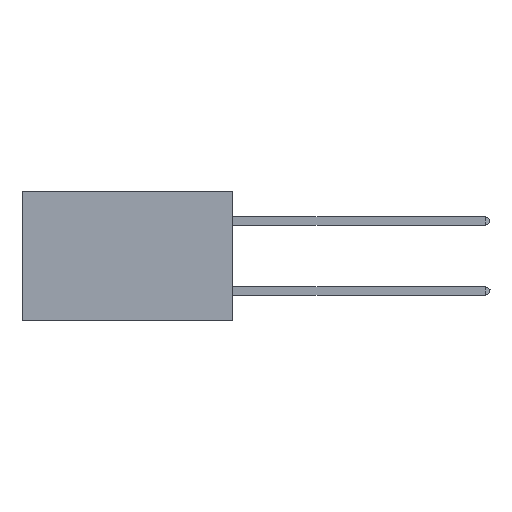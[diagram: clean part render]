
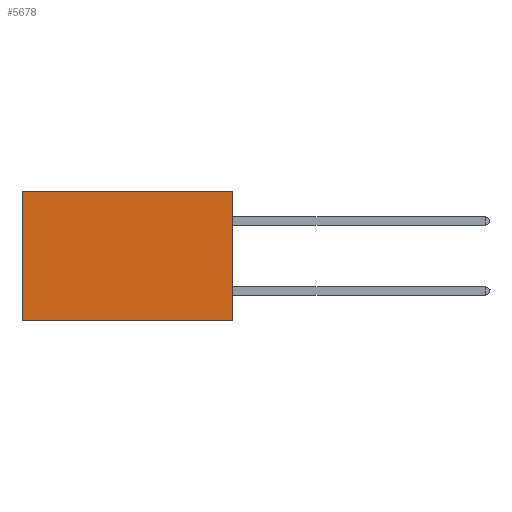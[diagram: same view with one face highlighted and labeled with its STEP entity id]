
A CAD part, left-side view. The second image highlights one B-rep face of the part: STEP entity #5678.
In plain terms, the highlighted planar face has unit normal (-1, 0, 0).
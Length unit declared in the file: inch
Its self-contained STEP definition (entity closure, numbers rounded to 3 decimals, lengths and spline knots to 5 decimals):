
#135 = EDGE_CURVE ( 'NONE', #30782, #31459, #36376, .T. ) ;
#1644 = CARTESIAN_POINT ( 'NONE',  ( 0.2875, 0.6, 0. ) ) ;
#2100 = EDGE_CURVE ( 'NONE', #31459, #12712, #21118, .T. ) ;
#2387 = PLANE ( 'NONE',  #11095 ) ;
#5678 = ADVANCED_FACE ( 'NONE', ( #24798 ), #2387, .F. ) ;
#5792 = DIRECTION ( 'NONE',  ( 0., 0., -1. ) ) ;
#11095 = AXIS2_PLACEMENT_3D ( 'NONE', #22445, #25811, #5792 ) ;
#11371 = CARTESIAN_POINT ( 'NONE',  ( 0.2875, 0., 0. ) ) ;
#11393 = DIRECTION ( 'NONE',  ( 0., 0., -1. ) ) ;
#12178 = ORIENTED_EDGE ( 'NONE', *, *, #22029, .F. ) ;
#12267 = VECTOR ( 'NONE', #35569, 39.37008 ) ;
#12465 = VECTOR ( 'NONE', #22555, 39.37008 ) ;
#12712 = VERTEX_POINT ( 'NONE', #16471 ) ;
#16471 = CARTESIAN_POINT ( 'NONE',  ( 0.2875, 0.6, -0.37 ) ) ;
#18681 = VECTOR ( 'NONE', #29084, 39.37008 ) ;
#21118 = LINE ( 'NONE', #1644, #12267 ) ;
#22029 = EDGE_CURVE ( 'NONE', #30782, #32341, #35610, .T. ) ;
#22166 = CARTESIAN_POINT ( 'NONE',  ( 0.2875, 0., -0.37 ) ) ;
#22445 = CARTESIAN_POINT ( 'NONE',  ( 0.2875, 0., 0. ) ) ;
#22555 = DIRECTION ( 'NONE',  ( 0., 1., 0. ) ) ;
#24640 = EDGE_CURVE ( 'NONE', #32341, #12712, #37960, .T. ) ;
#24728 = CARTESIAN_POINT ( 'NONE',  ( 0.2875, 0.6, 0. ) ) ;
#24798 = FACE_OUTER_BOUND ( 'NONE', #40482, .T. ) ;
#25811 = DIRECTION ( 'NONE',  ( 1., 0., 0. ) ) ;
#26782 = VECTOR ( 'NONE', #11393, 39.37008 ) ;
#29084 = DIRECTION ( 'NONE',  ( 0., 1., 0. ) ) ;
#30782 = VERTEX_POINT ( 'NONE', #11371 ) ;
#31304 = CARTESIAN_POINT ( 'NONE',  ( 0.2875, 0., 0. ) ) ;
#31459 = VERTEX_POINT ( 'NONE', #24728 ) ;
#32341 = VERTEX_POINT ( 'NONE', #22166 ) ;
#32787 = ORIENTED_EDGE ( 'NONE', *, *, #2100, .T. ) ;
#33405 = ORIENTED_EDGE ( 'NONE', *, *, #135, .T. ) ;
#35569 = DIRECTION ( 'NONE',  ( 0., 0., -1. ) ) ;
#35610 = LINE ( 'NONE', #31304, #26782 ) ;
#36376 = LINE ( 'NONE', #38009, #18681 ) ;
#37960 = LINE ( 'NONE', #39104, #12465 ) ;
#38009 = CARTESIAN_POINT ( 'NONE',  ( 0.2875, 0., 0. ) ) ;
#39104 = CARTESIAN_POINT ( 'NONE',  ( 0.2875, 0., -0.37 ) ) ;
#40482 = EDGE_LOOP ( 'NONE', ( #32787, #41548, #12178, #33405 ) ) ;
#41548 = ORIENTED_EDGE ( 'NONE', *, *, #24640, .F. ) ;
